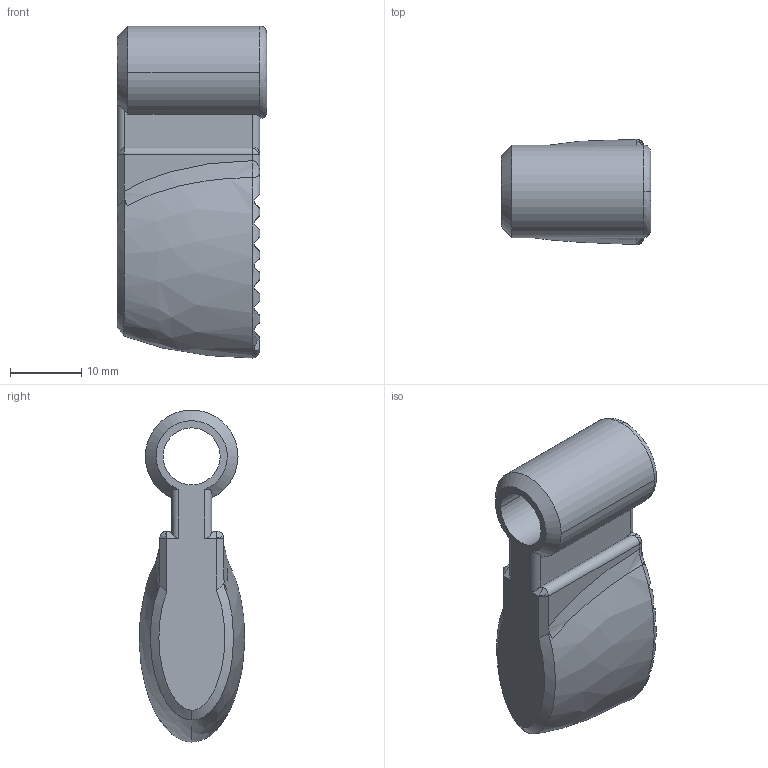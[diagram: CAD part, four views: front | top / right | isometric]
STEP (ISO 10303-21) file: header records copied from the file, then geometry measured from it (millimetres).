
FILE_DESCRIPTION (( 'STEP AP203' ), '1' );
FILE_NAME ('MOD9_V3_Charging_Handle.STEP', '2020-12-23T17:50:06', ( '' ), ( '' ), 'SwSTEP 2.0', 'SolidWorks 2019', '' );
FILE_SCHEMA (( 'CONFIG_CONTROL_DESIGN' ));
Length unit declared in the file: millimetre
Products named in the file (1): MOD9_V3_Charging_Handle
Bounding box: 21 x 14.76 x 46.57 mm (x, y, z)
Volume: 8310.3 mm3; surface area: 3556 mm2
Topology: 1 solids, 1 shells, 182 faces, 497 edges, 321 vertices
Faces by surface type: plane 147, bspline 17, cylinder 15, cone 3
Entity records: 6970 total; most frequent: CARTESIAN_POINT 2604, ORIENTED_EDGE 978, DIRECTION 734, EDGE_CURVE 489, LINE 334, VECTOR 334, VERTEX_POINT 321, AXIS2_PLACEMENT_3D 200
